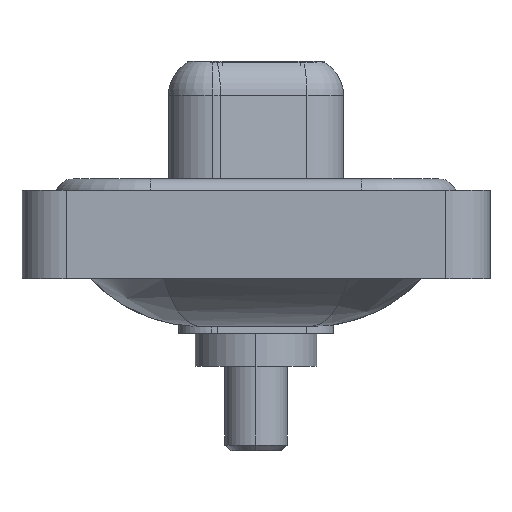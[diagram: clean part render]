
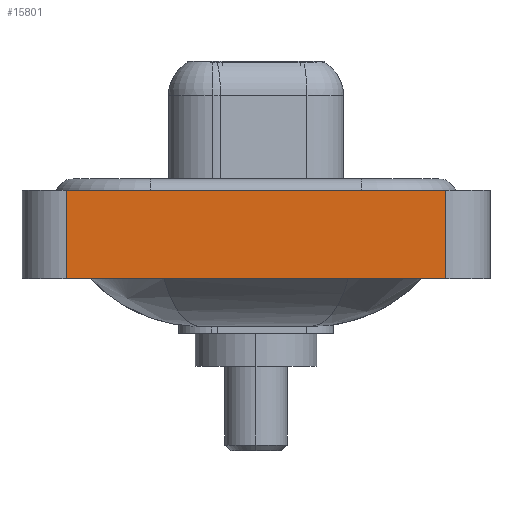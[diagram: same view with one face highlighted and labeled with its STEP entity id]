
A CAD part, left-side view. The second image highlights one B-rep face of the part: STEP entity #15801.
In plain terms, the highlighted planar face has unit normal (-1, 0, 0).
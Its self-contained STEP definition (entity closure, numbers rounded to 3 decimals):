
#816 = VECTOR ( 'NONE', #4483, 1000. ) ;
#1001 = CARTESIAN_POINT ( 'NONE',  ( -7.3, -8.55, -3.6 ) ) ;
#2004 = CARTESIAN_POINT ( 'NONE',  ( -7.3, 8.55, 0.4 ) ) ;
#2449 = EDGE_CURVE ( 'NONE', #15146, #10142, #7441, .T. ) ;
#2459 = CARTESIAN_POINT ( 'NONE',  ( -7.3, -8.55, -3.6 ) ) ;
#2846 = EDGE_LOOP ( 'NONE', ( #11007, #6000, #8515, #12323 ) ) ;
#3847 = DIRECTION ( 'NONE',  ( -1., 0., 0. ) ) ;
#4483 = DIRECTION ( 'NONE',  ( 0., 0., 1. ) ) ;
#5308 = VERTEX_POINT ( 'NONE', #2004 ) ;
#5616 = VECTOR ( 'NONE', #10836, 1000. ) ;
#6000 = ORIENTED_EDGE ( 'NONE', *, *, #15127, .F. ) ;
#6217 = DIRECTION ( 'NONE',  ( 0., -1., 0. ) ) ;
#7102 = CARTESIAN_POINT ( 'NONE',  ( -7.3, -8.55, -3.6 ) ) ;
#7258 = EDGE_CURVE ( 'NONE', #10142, #10188, #12018, .T. ) ;
#7280 = PLANE ( 'NONE',  #8321 ) ;
#7441 = LINE ( 'NONE', #9632, #5616 ) ;
#8321 = AXIS2_PLACEMENT_3D ( 'NONE', #2459, #3847, #13649 ) ;
#8515 = ORIENTED_EDGE ( 'NONE', *, *, #11246, .F. ) ;
#8949 = VECTOR ( 'NONE', #6217, 1000. ) ;
#9632 = CARTESIAN_POINT ( 'NONE',  ( -7.3, -8.55, -3.6 ) ) ;
#10142 = VERTEX_POINT ( 'NONE', #7102 ) ;
#10188 = VERTEX_POINT ( 'NONE', #11050 ) ;
#10746 = VECTOR ( 'NONE', #14259, 1000. ) ;
#10836 = DIRECTION ( 'NONE',  ( 0., -1., 0. ) ) ;
#11007 = ORIENTED_EDGE ( 'NONE', *, *, #7258, .T. ) ;
#11050 = CARTESIAN_POINT ( 'NONE',  ( -7.3, -8.55, 0.4 ) ) ;
#11246 = EDGE_CURVE ( 'NONE', #15146, #5308, #11628, .T. ) ;
#11450 = CARTESIAN_POINT ( 'NONE',  ( -7.3, -8.55, 0.4 ) ) ;
#11628 = LINE ( 'NONE', #14111, #816 ) ;
#12018 = LINE ( 'NONE', #1001, #10746 ) ;
#12323 = ORIENTED_EDGE ( 'NONE', *, *, #2449, .T. ) ;
#13649 = DIRECTION ( 'NONE',  ( 0., 0., 1. ) ) ;
#14111 = CARTESIAN_POINT ( 'NONE',  ( -7.3, 8.55, -3.6 ) ) ;
#14259 = DIRECTION ( 'NONE',  ( 0., 0., 1. ) ) ;
#14801 = CARTESIAN_POINT ( 'NONE',  ( -7.3, 8.55, -3.6 ) ) ;
#15127 = EDGE_CURVE ( 'NONE', #5308, #10188, #15134, .T. ) ;
#15134 = LINE ( 'NONE', #11450, #8949 ) ;
#15146 = VERTEX_POINT ( 'NONE', #14801 ) ;
#15801 = ADVANCED_FACE ( 'NONE', ( #15866 ), #7280, .T. ) ;
#15866 = FACE_OUTER_BOUND ( 'NONE', #2846, .T. ) ;
